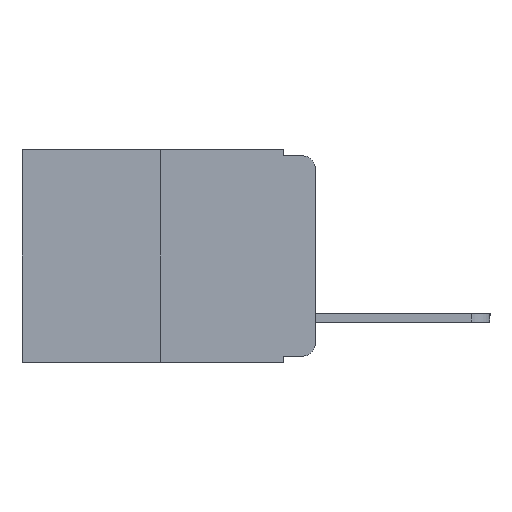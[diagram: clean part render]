
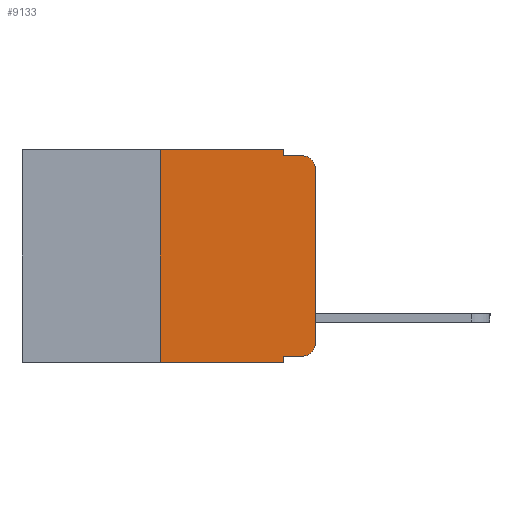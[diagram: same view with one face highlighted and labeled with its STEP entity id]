
A CAD part, left-side view. The second image highlights one B-rep face of the part: STEP entity #9133.
In plain terms, the highlighted planar face has unit normal (-1, 0, 0).
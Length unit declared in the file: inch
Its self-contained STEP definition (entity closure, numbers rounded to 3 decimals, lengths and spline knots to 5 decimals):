
#6 = ORIENTED_EDGE ( 'NONE', *, *, #6616, .T. ) ;
#267 = VERTEX_POINT ( 'NONE', #782 ) ;
#782 = CARTESIAN_POINT ( 'NONE',  ( 0., 0.25, 0. ) ) ;
#1228 = EDGE_CURVE ( 'NONE', #3986, #9929, #9000, .T. ) ;
#1359 = AXIS2_PLACEMENT_3D ( 'NONE', #9449, #13842, #14512 ) ;
#1607 = CARTESIAN_POINT ( 'NONE',  ( 0., 0.051, -0.343 ) ) ;
#1685 = VECTOR ( 'NONE', #3089, 39.37008 ) ;
#2080 = CARTESIAN_POINT ( 'NONE',  ( 0., 0.051, 0. ) ) ;
#2179 = LINE ( 'NONE', #17353, #1685 ) ;
#2313 = EDGE_CURVE ( 'NONE', #11945, #3986, #2179, .T. ) ;
#3089 = DIRECTION ( 'NONE',  ( 0., 0., -1. ) ) ;
#3116 = CARTESIAN_POINT ( 'NONE',  ( 0., 0.02, -0.01 ) ) ;
#3350 = ORIENTED_EDGE ( 'NONE', *, *, #5539, .T. ) ;
#3374 = EDGE_CURVE ( 'NONE', #6821, #267, #11075, .T. ) ;
#3871 = ORIENTED_EDGE ( 'NONE', *, *, #18442, .T. ) ;
#3986 = VERTEX_POINT ( 'NONE', #6705 ) ;
#4472 = EDGE_CURVE ( 'NONE', #5970, #16173, #9069, .T. ) ;
#5539 = EDGE_CURVE ( 'NONE', #5970, #15308, #14855, .T. ) ;
#5616 = VECTOR ( 'NONE', #9095, 39.37008 ) ;
#5822 = DIRECTION ( 'NONE',  ( 0., -1., 0. ) ) ;
#5842 = FACE_OUTER_BOUND ( 'NONE', #15457, .T. ) ;
#5970 = VERTEX_POINT ( 'NONE', #13070 ) ;
#6097 = VECTOR ( 'NONE', #7815, 39.37008 ) ;
#6547 = CARTESIAN_POINT ( 'NONE',  ( 0., 0.25, -0.343 ) ) ;
#6566 = DIRECTION ( 'NONE',  ( -1., 0., 0. ) ) ;
#6616 = EDGE_CURVE ( 'NONE', #15308, #16781, #7734, .T. ) ;
#6705 = CARTESIAN_POINT ( 'NONE',  ( 0., 0.051, -0.01 ) ) ;
#6821 = VERTEX_POINT ( 'NONE', #6547 ) ;
#7122 = CARTESIAN_POINT ( 'NONE',  ( 0., 0.473, -0.343 ) ) ;
#7547 = CARTESIAN_POINT ( 'NONE',  ( 0., 0., 0. ) ) ;
#7734 = CIRCLE ( 'NONE', #11668, 0.02 ) ;
#7815 = DIRECTION ( 'NONE',  ( 0., -1., 0. ) ) ;
#8597 = CARTESIAN_POINT ( 'NONE',  ( 0., 0.051, 0. ) ) ;
#8920 = CARTESIAN_POINT ( 'NONE',  ( 0., 0.02, -0.313 ) ) ;
#8963 = CARTESIAN_POINT ( 'NONE',  ( 0., 0.02, -0.333 ) ) ;
#9000 = LINE ( 'NONE', #12092, #16326 ) ;
#9069 = LINE ( 'NONE', #2080, #16865 ) ;
#9095 = DIRECTION ( 'NONE',  ( 0., 0., 1. ) ) ;
#9120 = ORIENTED_EDGE ( 'NONE', *, *, #1228, .F. ) ;
#9133 = ADVANCED_FACE ( 'NONE', ( #5842 ), #12755, .F. ) ;
#9449 = CARTESIAN_POINT ( 'NONE',  ( 0., 0.473, 0. ) ) ;
#9559 = DIRECTION ( 'NONE',  ( 0., -1., 0. ) ) ;
#9929 = VERTEX_POINT ( 'NONE', #3116 ) ;
#10052 = ORIENTED_EDGE ( 'NONE', *, *, #13681, .T. ) ;
#10489 = DIRECTION ( 'NONE',  ( 0., 0., -1. ) ) ;
#10598 = VECTOR ( 'NONE', #19078, 39.37008 ) ;
#10717 = VECTOR ( 'NONE', #9559, 39.37008 ) ;
#11017 = CARTESIAN_POINT ( 'NONE',  ( 0., 0.051, -0.333 ) ) ;
#11075 = LINE ( 'NONE', #20362, #10598 ) ;
#11455 = ORIENTED_EDGE ( 'NONE', *, *, #18564, .F. ) ;
#11668 = AXIS2_PLACEMENT_3D ( 'NONE', #8920, #19713, #10489 ) ;
#11945 = VERTEX_POINT ( 'NONE', #8597 ) ;
#12092 = CARTESIAN_POINT ( 'NONE',  ( 0., 0.051, -0.01 ) ) ;
#12669 = LINE ( 'NONE', #7122, #17765 ) ;
#12755 = PLANE ( 'NONE',  #1359 ) ;
#12880 = CARTESIAN_POINT ( 'NONE',  ( 0., 0., -0.313 ) ) ;
#13070 = CARTESIAN_POINT ( 'NONE',  ( 0., 0.051, -0.333 ) ) ;
#13206 = ORIENTED_EDGE ( 'NONE', *, *, #3374, .F. ) ;
#13681 = EDGE_CURVE ( 'NONE', #6821, #16173, #12669, .T. ) ;
#13842 = DIRECTION ( 'NONE',  ( 1., 0., 0. ) ) ;
#14245 = DIRECTION ( 'NONE',  ( 0., 0., -1. ) ) ;
#14512 = DIRECTION ( 'NONE',  ( 0., 0., -1. ) ) ;
#14634 = CARTESIAN_POINT ( 'NONE',  ( 0., 0., -0.03 ) ) ;
#14855 = LINE ( 'NONE', #11017, #10717 ) ;
#14885 = DIRECTION ( 'NONE',  ( 0., -1., 0. ) ) ;
#15308 = VERTEX_POINT ( 'NONE', #8963 ) ;
#15457 = EDGE_LOOP ( 'NONE', ( #3871, #19724, #9120, #18448, #11455, #13206, #10052, #17120, #3350, #6 ) ) ;
#15614 = CIRCLE ( 'NONE', #18808, 0.02 ) ;
#15954 = CARTESIAN_POINT ( 'NONE',  ( 0., 0.02, -0.03 ) ) ;
#16173 = VERTEX_POINT ( 'NONE', #1607 ) ;
#16326 = VECTOR ( 'NONE', #5822, 39.37008 ) ;
#16781 = VERTEX_POINT ( 'NONE', #12880 ) ;
#16865 = VECTOR ( 'NONE', #14245, 39.37008 ) ;
#17120 = ORIENTED_EDGE ( 'NONE', *, *, #4472, .F. ) ;
#17353 = CARTESIAN_POINT ( 'NONE',  ( 0., 0.051, 0. ) ) ;
#17487 = DIRECTION ( 'NONE',  ( 0., 0., -1. ) ) ;
#17765 = VECTOR ( 'NONE', #14885, 39.37008 ) ;
#18063 = LINE ( 'NONE', #7547, #5616 ) ;
#18442 = EDGE_CURVE ( 'NONE', #16781, #19624, #18063, .T. ) ;
#18448 = ORIENTED_EDGE ( 'NONE', *, *, #2313, .F. ) ;
#18497 = LINE ( 'NONE', #18542, #6097 ) ;
#18542 = CARTESIAN_POINT ( 'NONE',  ( 0., 0.473, 0. ) ) ;
#18564 = EDGE_CURVE ( 'NONE', #267, #11945, #18497, .T. ) ;
#18808 = AXIS2_PLACEMENT_3D ( 'NONE', #15954, #6566, #17487 ) ;
#19078 = DIRECTION ( 'NONE',  ( 0., 0., 1. ) ) ;
#19479 = EDGE_CURVE ( 'NONE', #19624, #9929, #15614, .T. ) ;
#19624 = VERTEX_POINT ( 'NONE', #14634 ) ;
#19713 = DIRECTION ( 'NONE',  ( -1., 0., 0. ) ) ;
#19724 = ORIENTED_EDGE ( 'NONE', *, *, #19479, .T. ) ;
#20362 = CARTESIAN_POINT ( 'NONE',  ( 0., 0.25, 0. ) ) ;
